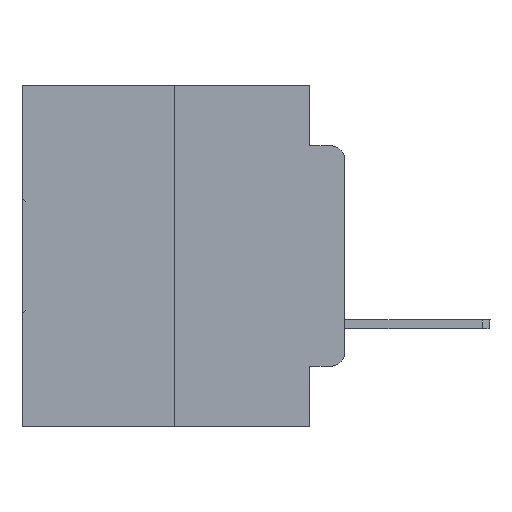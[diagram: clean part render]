
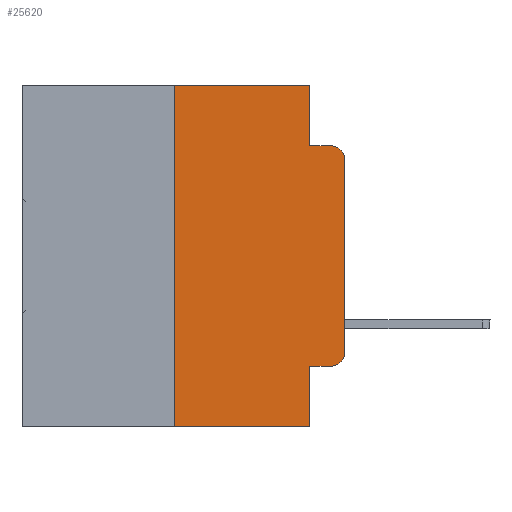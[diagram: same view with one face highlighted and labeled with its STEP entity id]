
A CAD part, left-side view. The second image highlights one B-rep face of the part: STEP entity #25620.
In plain terms, the highlighted planar face has unit normal (-1, 0, 0).
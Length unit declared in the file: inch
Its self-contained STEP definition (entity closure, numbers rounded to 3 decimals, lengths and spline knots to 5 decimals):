
#268 = CARTESIAN_POINT ( 'NONE',  ( 0., 0.02, -0.0885 ) ) ;
#370 = CARTESIAN_POINT ( 'NONE',  ( 0., 0., -0.1085 ) ) ;
#508 = EDGE_CURVE ( 'NONE', #5809, #20701, #24040, .T. ) ;
#637 = DIRECTION ( 'NONE',  ( -1., 0., 0. ) ) ;
#674 = EDGE_CURVE ( 'NONE', #19730, #8380, #5927, .T. ) ;
#683 = VECTOR ( 'NONE', #19131, 39.37008 ) ;
#795 = VECTOR ( 'NONE', #15129, 39.37008 ) ;
#893 = LINE ( 'NONE', #28595, #10686 ) ;
#928 = VERTEX_POINT ( 'NONE', #7570 ) ;
#983 = EDGE_CURVE ( 'NONE', #928, #28394, #23401, .T. ) ;
#1037 = VERTEX_POINT ( 'NONE', #24298 ) ;
#1309 = CARTESIAN_POINT ( 'NONE',  ( 0., 0.051, 0. ) ) ;
#1973 = LINE ( 'NONE', #29511, #15875 ) ;
#3461 = DIRECTION ( 'NONE',  ( 0., 0., -1. ) ) ;
#5809 = VERTEX_POINT ( 'NONE', #370 ) ;
#5927 = LINE ( 'NONE', #10331, #27049 ) ;
#6451 = EDGE_CURVE ( 'NONE', #28394, #29900, #12879, .T. ) ;
#6487 = ORIENTED_EDGE ( 'NONE', *, *, #13963, .F. ) ;
#6676 = VECTOR ( 'NONE', #10567, 39.37008 ) ;
#6796 = VECTOR ( 'NONE', #3461, 39.37008 ) ;
#7044 = CARTESIAN_POINT ( 'NONE',  ( 0., 0.473, 0. ) ) ;
#7570 = CARTESIAN_POINT ( 'NONE',  ( 0., 0.051, -0.4115 ) ) ;
#7892 = DIRECTION ( 'NONE',  ( 0., 0., 1. ) ) ;
#8380 = VERTEX_POINT ( 'NONE', #25251 ) ;
#8429 = LINE ( 'NONE', #26855, #795 ) ;
#9288 = DIRECTION ( 'NONE',  ( -1., 0., 0. ) ) ;
#9433 = LINE ( 'NONE', #27857, #18091 ) ;
#9692 = CARTESIAN_POINT ( 'NONE',  ( 0., 0.051, -0.4115 ) ) ;
#10075 = DIRECTION ( 'NONE',  ( 0., 0., -1. ) ) ;
#10331 = CARTESIAN_POINT ( 'NONE',  ( 0., 0.051, 0. ) ) ;
#10567 = DIRECTION ( 'NONE',  ( 0., 0., 1. ) ) ;
#10686 = VECTOR ( 'NONE', #7892, 39.37008 ) ;
#10804 = ORIENTED_EDGE ( 'NONE', *, *, #508, .T. ) ;
#11457 = CARTESIAN_POINT ( 'NONE',  ( 0., 0.02, -0.4115 ) ) ;
#12248 = AXIS2_PLACEMENT_3D ( 'NONE', #7044, #16320, #16626 ) ;
#12581 = LINE ( 'NONE', #1309, #6796 ) ;
#12617 = DIRECTION ( 'NONE',  ( 0., 0., -1. ) ) ;
#12728 = CARTESIAN_POINT ( 'NONE',  ( 0., 0.25, 0. ) ) ;
#12879 = CIRCLE ( 'NONE', #19707, 0.02 ) ;
#13427 = ORIENTED_EDGE ( 'NONE', *, *, #26125, .F. ) ;
#13654 = ORIENTED_EDGE ( 'NONE', *, *, #16985, .T. ) ;
#13963 = EDGE_CURVE ( 'NONE', #928, #17044, #12581, .T. ) ;
#14030 = VERTEX_POINT ( 'NONE', #12728 ) ;
#14681 = ORIENTED_EDGE ( 'NONE', *, *, #22066, .T. ) ;
#15129 = DIRECTION ( 'NONE',  ( 0., -1., 0. ) ) ;
#15130 = CARTESIAN_POINT ( 'NONE',  ( 0., 0.25, 0. ) ) ;
#15809 = ORIENTED_EDGE ( 'NONE', *, *, #983, .T. ) ;
#15875 = VECTOR ( 'NONE', #24928, 39.37008 ) ;
#16320 = DIRECTION ( 'NONE',  ( 1., 0., 0. ) ) ;
#16329 = CARTESIAN_POINT ( 'NONE',  ( 0., 0.051, 0. ) ) ;
#16626 = DIRECTION ( 'NONE',  ( 0., 0., -1. ) ) ;
#16896 = DIRECTION ( 'NONE',  ( 0., -1., 0. ) ) ;
#16985 = EDGE_CURVE ( 'NONE', #1037, #17044, #8429, .T. ) ;
#17044 = VERTEX_POINT ( 'NONE', #19042 ) ;
#17412 = EDGE_CURVE ( 'NONE', #14030, #19730, #1973, .T. ) ;
#17540 = CARTESIAN_POINT ( 'NONE',  ( 0., 0., -0.3915 ) ) ;
#17968 = ORIENTED_EDGE ( 'NONE', *, *, #29426, .F. ) ;
#18091 = VECTOR ( 'NONE', #16896, 39.37008 ) ;
#18325 = ORIENTED_EDGE ( 'NONE', *, *, #17412, .F. ) ;
#18614 = FACE_OUTER_BOUND ( 'NONE', #23635, .T. ) ;
#18663 = ORIENTED_EDGE ( 'NONE', *, *, #6451, .T. ) ;
#19042 = CARTESIAN_POINT ( 'NONE',  ( 0., 0.051, -0.5 ) ) ;
#19131 = DIRECTION ( 'NONE',  ( 0., -1., 0. ) ) ;
#19417 = LINE ( 'NONE', #15130, #6676 ) ;
#19707 = AXIS2_PLACEMENT_3D ( 'NONE', #28795, #637, #10075 ) ;
#19730 = VERTEX_POINT ( 'NONE', #16329 ) ;
#20701 = VERTEX_POINT ( 'NONE', #268 ) ;
#22066 = EDGE_CURVE ( 'NONE', #29900, #5809, #893, .T. ) ;
#23401 = LINE ( 'NONE', #9692, #683 ) ;
#23635 = EDGE_LOOP ( 'NONE', ( #14681, #10804, #13427, #28753, #18325, #17968, #13654, #6487, #15809, #18663 ) ) ;
#24040 = CIRCLE ( 'NONE', #24544, 0.02 ) ;
#24298 = CARTESIAN_POINT ( 'NONE',  ( 0., 0.25, -0.5 ) ) ;
#24544 = AXIS2_PLACEMENT_3D ( 'NONE', #25864, #9288, #27848 ) ;
#24928 = DIRECTION ( 'NONE',  ( 0., -1., 0. ) ) ;
#25251 = CARTESIAN_POINT ( 'NONE',  ( 0., 0.051, -0.0885 ) ) ;
#25620 = ADVANCED_FACE ( 'NONE', ( #18614 ), #27889, .F. ) ;
#25864 = CARTESIAN_POINT ( 'NONE',  ( 0., 0.02, -0.1085 ) ) ;
#26125 = EDGE_CURVE ( 'NONE', #8380, #20701, #9433, .T. ) ;
#26855 = CARTESIAN_POINT ( 'NONE',  ( 0., 0.473, -0.5 ) ) ;
#27049 = VECTOR ( 'NONE', #12617, 39.37008 ) ;
#27848 = DIRECTION ( 'NONE',  ( 0., 0., -1. ) ) ;
#27857 = CARTESIAN_POINT ( 'NONE',  ( 0., 0.051, -0.0885 ) ) ;
#27889 = PLANE ( 'NONE',  #12248 ) ;
#28394 = VERTEX_POINT ( 'NONE', #11457 ) ;
#28595 = CARTESIAN_POINT ( 'NONE',  ( 0., 0., 0. ) ) ;
#28753 = ORIENTED_EDGE ( 'NONE', *, *, #674, .F. ) ;
#28795 = CARTESIAN_POINT ( 'NONE',  ( 0., 0.02, -0.3915 ) ) ;
#29426 = EDGE_CURVE ( 'NONE', #1037, #14030, #19417, .T. ) ;
#29511 = CARTESIAN_POINT ( 'NONE',  ( 0., 0.473, 0. ) ) ;
#29900 = VERTEX_POINT ( 'NONE', #17540 ) ;
